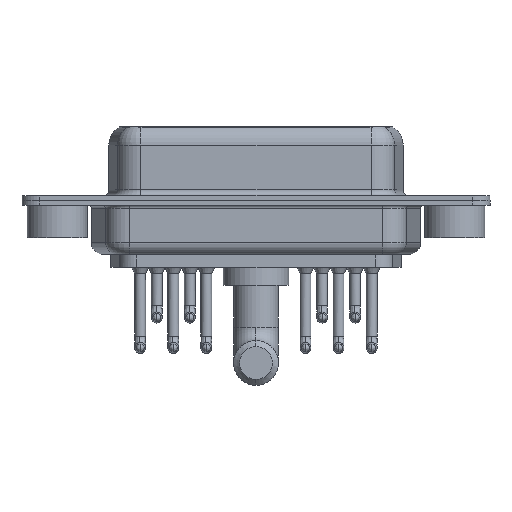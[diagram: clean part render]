
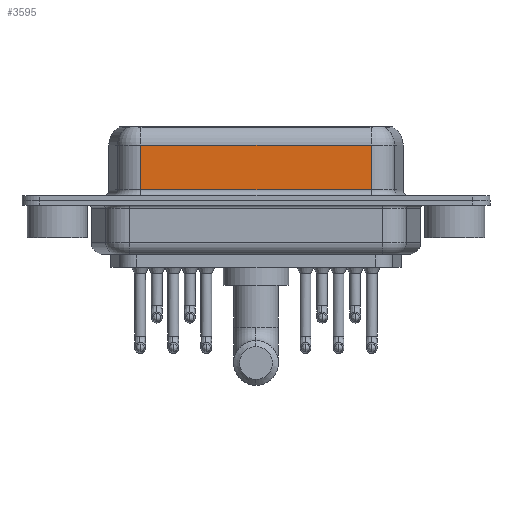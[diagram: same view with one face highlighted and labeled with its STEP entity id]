
A CAD part, front view. The second image highlights one B-rep face of the part: STEP entity #3595.
In plain terms, the highlighted planar face has unit normal (0, -1, 0).
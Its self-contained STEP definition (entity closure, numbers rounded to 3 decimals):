
#356 = LINE ( 'NONE', #13218, #5900 ) ;
#1364 = VECTOR ( 'NONE', #4737, 1000. ) ;
#1508 = PLANE ( 'NONE',  #5201 ) ;
#1512 = VECTOR ( 'NONE', #9913, 1000. ) ;
#1697 = FACE_OUTER_BOUND ( 'NONE', #1724, .T. ) ;
#1724 = EDGE_LOOP ( 'NONE', ( #3603, #10601, #4925, #8696 ) ) ;
#1964 = DIRECTION ( 'NONE',  ( 0., 0., 1. ) ) ;
#3221 = LINE ( 'NONE', #13417, #1364 ) ;
#3595 = ADVANCED_FACE ( 'NONE', ( #1697 ), #1508, .F. ) ;
#3603 = ORIENTED_EDGE ( 'NONE', *, *, #15384, .F. ) ;
#4010 = CARTESIAN_POINT ( 'NONE',  ( 26.287, -3.95, 4.65 ) ) ;
#4163 = CARTESIAN_POINT ( 'NONE',  ( 26.287, -3.95, 0.9 ) ) ;
#4737 = DIRECTION ( 'NONE',  ( 0., 0., -1. ) ) ;
#4766 = VERTEX_POINT ( 'NONE', #4010 ) ;
#4902 = DIRECTION ( 'NONE',  ( 0., 1., 0. ) ) ;
#4925 = ORIENTED_EDGE ( 'NONE', *, *, #16964, .T. ) ;
#4967 = VERTEX_POINT ( 'NONE', #14873 ) ;
#5201 = AXIS2_PLACEMENT_3D ( 'NONE', #7992, #4902, #1964 ) ;
#5715 = EDGE_CURVE ( 'NONE', #4766, #8407, #18660, .T. ) ;
#5900 = VECTOR ( 'NONE', #10276, 1000. ) ;
#7992 = CARTESIAN_POINT ( 'NONE',  ( 26.287, -3.95, 6.4 ) ) ;
#8407 = VERTEX_POINT ( 'NONE', #18588 ) ;
#8696 = ORIENTED_EDGE ( 'NONE', *, *, #11724, .T. ) ;
#9184 = VECTOR ( 'NONE', #10195, 1000. ) ;
#9913 = DIRECTION ( 'NONE',  ( 1., 0., 0. ) ) ;
#10195 = DIRECTION ( 'NONE',  ( -1., 0., 0. ) ) ;
#10276 = DIRECTION ( 'NONE',  ( 0., 0., -1. ) ) ;
#10601 = ORIENTED_EDGE ( 'NONE', *, *, #5715, .T. ) ;
#10616 = CARTESIAN_POINT ( 'NONE',  ( 26.287, -3.95, 0.9 ) ) ;
#11724 = EDGE_CURVE ( 'NONE', #4967, #17418, #18663, .T. ) ;
#13218 = CARTESIAN_POINT ( 'NONE',  ( 26.287, -3.95, 6.4 ) ) ;
#13417 = CARTESIAN_POINT ( 'NONE',  ( 7.013, -3.95, 6.4 ) ) ;
#14873 = CARTESIAN_POINT ( 'NONE',  ( 7.013, -3.95, 0.9 ) ) ;
#15384 = EDGE_CURVE ( 'NONE', #4766, #17418, #356, .T. ) ;
#15709 = CARTESIAN_POINT ( 'NONE',  ( 26.287, -3.95, 4.65 ) ) ;
#16964 = EDGE_CURVE ( 'NONE', #8407, #4967, #3221, .T. ) ;
#17418 = VERTEX_POINT ( 'NONE', #10616 ) ;
#18588 = CARTESIAN_POINT ( 'NONE',  ( 7.013, -3.95, 4.65 ) ) ;
#18660 = LINE ( 'NONE', #15709, #9184 ) ;
#18663 = LINE ( 'NONE', #4163, #1512 ) ;
